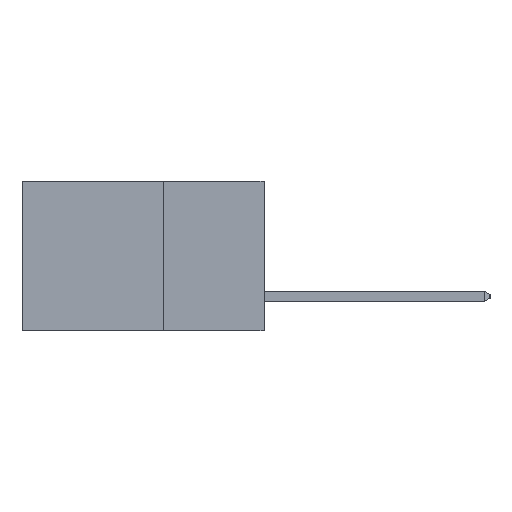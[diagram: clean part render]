
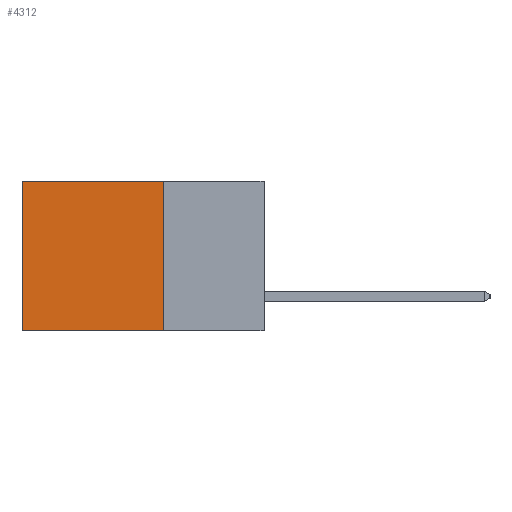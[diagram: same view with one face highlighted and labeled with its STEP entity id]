
A CAD part, left-side view. The second image highlights one B-rep face of the part: STEP entity #4312.
In plain terms, the highlighted planar face has unit normal (-1, 0, 0).
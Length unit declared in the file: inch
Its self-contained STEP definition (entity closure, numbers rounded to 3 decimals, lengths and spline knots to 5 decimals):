
#7 = ORIENTED_EDGE ( 'NONE', *, *, #645, .F. ) ;
#493 = LINE ( 'NONE', #8058, #2709 ) ;
#645 = EDGE_CURVE ( 'NONE', #6561, #8382, #8712, .T. ) ;
#698 = VERTEX_POINT ( 'NONE', #10937 ) ;
#1148 = VECTOR ( 'NONE', #4797, 39.37008 ) ;
#2250 = ORIENTED_EDGE ( 'NONE', *, *, #6807, .T. ) ;
#2368 = DIRECTION ( 'NONE',  ( 1., 0., 0. ) ) ;
#2447 = LINE ( 'NONE', #5951, #11679 ) ;
#2709 = VECTOR ( 'NONE', #8907, 39.37008 ) ;
#4312 = ADVANCED_FACE ( 'NONE', ( #9741 ), #8132, .F. ) ;
#4797 = DIRECTION ( 'NONE',  ( 0., 0., -1. ) ) ;
#5285 = ORIENTED_EDGE ( 'NONE', *, *, #5743, .T. ) ;
#5588 = LINE ( 'NONE', #10780, #9914 ) ;
#5743 = EDGE_CURVE ( 'NONE', #6561, #698, #2447, .T. ) ;
#5861 = EDGE_LOOP ( 'NONE', ( #2250, #9656, #7, #5285 ) ) ;
#5951 = CARTESIAN_POINT ( 'NONE',  ( 0.2615, 0.25, 0. ) ) ;
#6556 = AXIS2_PLACEMENT_3D ( 'NONE', #7257, #2368, #8985 ) ;
#6561 = VERTEX_POINT ( 'NONE', #10873 ) ;
#6574 = VERTEX_POINT ( 'NONE', #10366 ) ;
#6589 = DIRECTION ( 'NONE',  ( 0., 1., 0. ) ) ;
#6807 = EDGE_CURVE ( 'NONE', #698, #6574, #493, .T. ) ;
#7160 = EDGE_CURVE ( 'NONE', #8382, #6574, #5588, .T. ) ;
#7257 = CARTESIAN_POINT ( 'NONE',  ( 0.2615, 0.25, -0.37 ) ) ;
#7878 = CARTESIAN_POINT ( 'NONE',  ( 0.2615, 0.25, -0.37 ) ) ;
#8058 = CARTESIAN_POINT ( 'NONE',  ( 0.2615, 0.6, -0.37 ) ) ;
#8132 = PLANE ( 'NONE',  #6556 ) ;
#8382 = VERTEX_POINT ( 'NONE', #8417 ) ;
#8417 = CARTESIAN_POINT ( 'NONE',  ( 0.2615, 0.25, -0.37 ) ) ;
#8712 = LINE ( 'NONE', #7878, #1148 ) ;
#8907 = DIRECTION ( 'NONE',  ( 0., 0., -1. ) ) ;
#8985 = DIRECTION ( 'NONE',  ( 0., 0., -1. ) ) ;
#9435 = DIRECTION ( 'NONE',  ( 0., 1., 0. ) ) ;
#9656 = ORIENTED_EDGE ( 'NONE', *, *, #7160, .F. ) ;
#9741 = FACE_OUTER_BOUND ( 'NONE', #5861, .T. ) ;
#9914 = VECTOR ( 'NONE', #6589, 39.37008 ) ;
#10366 = CARTESIAN_POINT ( 'NONE',  ( 0.2615, 0.6, -0.37 ) ) ;
#10780 = CARTESIAN_POINT ( 'NONE',  ( 0.2615, 0.25, -0.37 ) ) ;
#10873 = CARTESIAN_POINT ( 'NONE',  ( 0.2615, 0.25, 0. ) ) ;
#10937 = CARTESIAN_POINT ( 'NONE',  ( 0.2615, 0.6, 0. ) ) ;
#11679 = VECTOR ( 'NONE', #9435, 39.37008 ) ;
